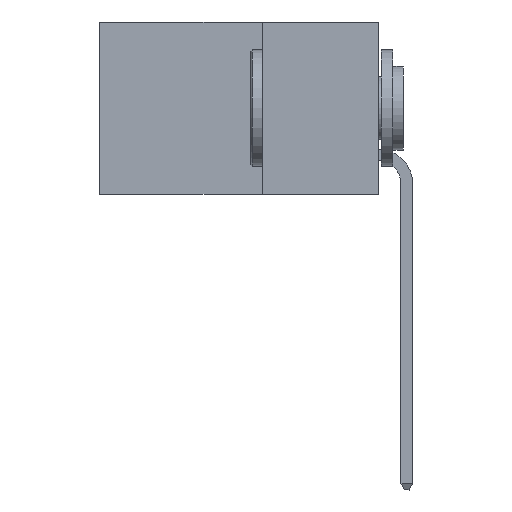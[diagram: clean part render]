
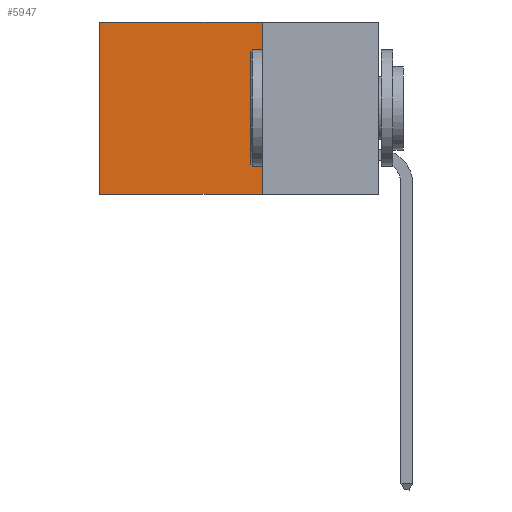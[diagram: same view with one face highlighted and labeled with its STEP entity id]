
A CAD part, left-side view. The second image highlights one B-rep face of the part: STEP entity #5947.
In plain terms, the highlighted planar face has unit normal (-1, 0, 0).
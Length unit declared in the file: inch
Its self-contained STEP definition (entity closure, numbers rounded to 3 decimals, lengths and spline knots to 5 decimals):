
#287 = EDGE_LOOP ( 'NONE', ( #6682, #7567, #1277, #5970 ) ) ;
#814 = DIRECTION ( 'NONE',  ( 0., 1., 0. ) ) ;
#917 = CARTESIAN_POINT ( 'NONE',  ( 0.2615, 0.25, 0. ) ) ;
#1277 = ORIENTED_EDGE ( 'NONE', *, *, #2828, .F. ) ;
#1320 = CARTESIAN_POINT ( 'NONE',  ( 0.2615, 0.25, -0.37 ) ) ;
#1364 = PLANE ( 'NONE',  #3884 ) ;
#1575 = VECTOR ( 'NONE', #2270, 39.37008 ) ;
#1619 = EDGE_CURVE ( 'NONE', #4142, #3814, #2600, .T. ) ;
#2270 = DIRECTION ( 'NONE',  ( 0., 0., -1. ) ) ;
#2600 = LINE ( 'NONE', #4789, #6083 ) ;
#2761 = EDGE_CURVE ( 'NONE', #8939, #5227, #8930, .T. ) ;
#2828 = EDGE_CURVE ( 'NONE', #8939, #4142, #7577, .T. ) ;
#2953 = FACE_OUTER_BOUND ( 'NONE', #287, .T. ) ;
#3542 = DIRECTION ( 'NONE',  ( 0., 0., -1. ) ) ;
#3620 = VECTOR ( 'NONE', #3625, 39.37008 ) ;
#3625 = DIRECTION ( 'NONE',  ( 0., 0., -1. ) ) ;
#3814 = VERTEX_POINT ( 'NONE', #3871 ) ;
#3871 = CARTESIAN_POINT ( 'NONE',  ( 0.2615, 0.6, -0.37 ) ) ;
#3884 = AXIS2_PLACEMENT_3D ( 'NONE', #8765, #4458, #3542 ) ;
#4142 = VERTEX_POINT ( 'NONE', #1320 ) ;
#4205 = CARTESIAN_POINT ( 'NONE',  ( 0.2615, 0.6, -0.37 ) ) ;
#4458 = DIRECTION ( 'NONE',  ( 1., 0., 0. ) ) ;
#4789 = CARTESIAN_POINT ( 'NONE',  ( 0.2615, 0.25, -0.37 ) ) ;
#5227 = VERTEX_POINT ( 'NONE', #5740 ) ;
#5740 = CARTESIAN_POINT ( 'NONE',  ( 0.2615, 0.6, 0. ) ) ;
#5791 = LINE ( 'NONE', #4205, #3620 ) ;
#5947 = ADVANCED_FACE ( 'NONE', ( #2953 ), #1364, .F. ) ;
#5970 = ORIENTED_EDGE ( 'NONE', *, *, #2761, .T. ) ;
#6083 = VECTOR ( 'NONE', #7685, 39.37008 ) ;
#6682 = ORIENTED_EDGE ( 'NONE', *, *, #7852, .T. ) ;
#6759 = CARTESIAN_POINT ( 'NONE',  ( 0.2615, 0.25, -0.37 ) ) ;
#7567 = ORIENTED_EDGE ( 'NONE', *, *, #1619, .F. ) ;
#7577 = LINE ( 'NONE', #6759, #1575 ) ;
#7685 = DIRECTION ( 'NONE',  ( 0., 1., 0. ) ) ;
#7852 = EDGE_CURVE ( 'NONE', #5227, #3814, #5791, .T. ) ;
#8765 = CARTESIAN_POINT ( 'NONE',  ( 0.2615, 0.25, -0.37 ) ) ;
#8930 = LINE ( 'NONE', #9070, #9283 ) ;
#8939 = VERTEX_POINT ( 'NONE', #917 ) ;
#9070 = CARTESIAN_POINT ( 'NONE',  ( 0.2615, 0.25, 0. ) ) ;
#9283 = VECTOR ( 'NONE', #814, 39.37008 ) ;
